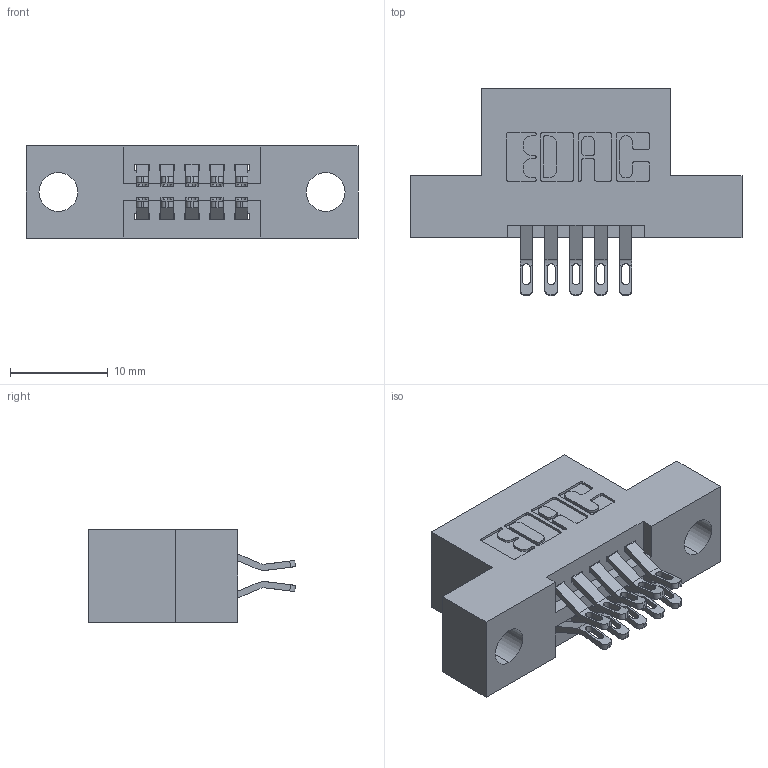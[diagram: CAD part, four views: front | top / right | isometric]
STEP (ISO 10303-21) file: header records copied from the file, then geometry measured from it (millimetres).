
FILE_DESCRIPTION (( 'STEP AP203' ), '1' );
FILE_NAME ('345-010-555-204.STEP', '2018-08-17T21:25:14', ( '' ), ( '' ), 'SwSTEP 2.0', 'SolidWorks 2016', '' );
FILE_SCHEMA (( 'CONFIG_CONTROL_DESIGN' ));
Length unit declared in the file: inch
Products named in the file (3): 345 Part_Flush Mounting Lugs - 0.156 Dia-TH; 345-292-001_555 Tail; 345-010-555-204
Assembly tree (11 placements, depth 2):
  345-010-555-204
    345 Part_Flush Mounting Lugs - 0.156 Dia-TH
    345-292-001_555 Tail  x10
Bounding box: 33.91 x 21.13 x 9.4 mm (x, y, z)
Volume: 2891.7 mm3; surface area: 3473.8 mm2
Topology: 11 solids, 11 shells, 686 faces, 2111 edges, 1406 vertices
Faces by surface type: plane 390, cylinder 296
Entity records: 9233 total; most frequent: CARTESIAN_POINT 1618, ORIENTED_EDGE 1522, DIRECTION 1441, EDGE_CURVE 761, VECTOR 589, LINE 589, VERTEX_POINT 506, AXIS2_PLACEMENT_3D 426
